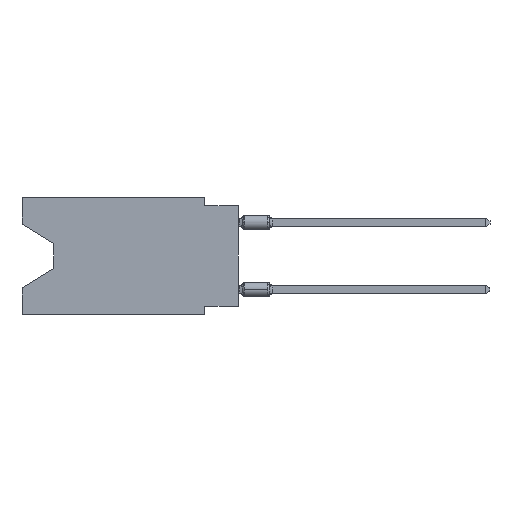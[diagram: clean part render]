
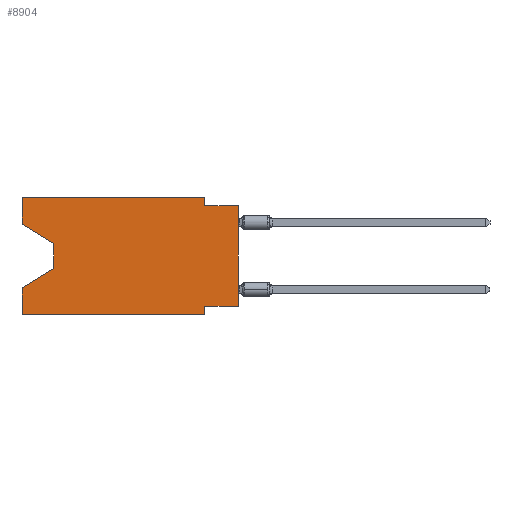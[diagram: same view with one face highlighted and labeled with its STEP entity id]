
A CAD part, left-side view. The second image highlights one B-rep face of the part: STEP entity #8904.
In plain terms, the highlighted planar face has unit normal (-1, 0, 0).
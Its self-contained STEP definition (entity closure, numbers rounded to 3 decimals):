
#585 = LINE ( 'NONE', #5144, #2630 ) ;
#1254 = EDGE_CURVE ( 'NONE', #11337, #13501, #20487, .T. ) ;
#1260 = EDGE_CURVE ( 'NONE', #18649, #28238, #6542, .T. ) ;
#2246 = EDGE_CURVE ( 'NONE', #20303, #17698, #585, .T. ) ;
#2630 = VECTOR ( 'NONE', #2946, 1000. ) ;
#2683 = VERTEX_POINT ( 'NONE', #18905 ) ;
#2846 = ORIENTED_EDGE ( 'NONE', *, *, #17076, .T. ) ;
#2946 = DIRECTION ( 'NONE',  ( 0., 0., 1. ) ) ;
#3536 = CARTESIAN_POINT ( 'NONE',  ( 0., 13.97, -3.505 ) ) ;
#3620 = VECTOR ( 'NONE', #18271, 1000. ) ;
#3776 = LINE ( 'NONE', #15995, #3787 ) ;
#3787 = VECTOR ( 'NONE', #20695, 1000. ) ;
#3843 = ORIENTED_EDGE ( 'NONE', *, *, #13008, .F. ) ;
#4056 = PLANE ( 'NONE',  #18541 ) ;
#5144 = CARTESIAN_POINT ( 'NONE',  ( 0., 16.383, 0. ) ) ;
#5709 = CARTESIAN_POINT ( 'NONE',  ( 0., 2.54, -8.89 ) ) ;
#5882 = CARTESIAN_POINT ( 'NONE',  ( 0., 16.383, -8.89 ) ) ;
#6039 = DIRECTION ( 'NONE',  ( 0., -1., 0. ) ) ;
#6542 = LINE ( 'NONE', #30690, #12105 ) ;
#6664 = LINE ( 'NONE', #25480, #3620 ) ;
#7456 = EDGE_CURVE ( 'NONE', #12397, #16086, #17240, .T. ) ;
#7503 = DIRECTION ( 'NONE',  ( 0., -1., 0. ) ) ;
#7618 = CARTESIAN_POINT ( 'NONE',  ( 0., 2.54, -8.255 ) ) ;
#7803 = DIRECTION ( 'NONE',  ( 0., 1., 0. ) ) ;
#8337 = CARTESIAN_POINT ( 'NONE',  ( 0., 0., -8.255 ) ) ;
#8385 = CARTESIAN_POINT ( 'NONE',  ( 0., 16.383, -2.038 ) ) ;
#8611 = LINE ( 'NONE', #29796, #20821 ) ;
#8904 = ADVANCED_FACE ( 'NONE', ( #23489 ), #4056, .F. ) ;
#10144 = CARTESIAN_POINT ( 'NONE',  ( 0., 0., -8.255 ) ) ;
#10667 = VERTEX_POINT ( 'NONE', #7618 ) ;
#10726 = DIRECTION ( 'NONE',  ( 0., 0., -1. ) ) ;
#10823 = DIRECTION ( 'NONE',  ( 0., 0., 1. ) ) ;
#10824 = EDGE_CURVE ( 'NONE', #28161, #13501, #24693, .T. ) ;
#10948 = EDGE_CURVE ( 'NONE', #28238, #28714, #6664, .T. ) ;
#11337 = VERTEX_POINT ( 'NONE', #8337 ) ;
#11439 = DIRECTION ( 'NONE',  ( 0., 0., -1. ) ) ;
#12105 = VECTOR ( 'NONE', #16103, 1000. ) ;
#12397 = VERTEX_POINT ( 'NONE', #30983 ) ;
#12553 = CARTESIAN_POINT ( 'NONE',  ( 0., 16.383, 0. ) ) ;
#12578 = ORIENTED_EDGE ( 'NONE', *, *, #13230, .F. ) ;
#12951 = CARTESIAN_POINT ( 'NONE',  ( 0., 2.54, -0.635 ) ) ;
#13008 = EDGE_CURVE ( 'NONE', #18649, #12397, #8611, .T. ) ;
#13088 = LINE ( 'NONE', #5709, #22534 ) ;
#13230 = EDGE_CURVE ( 'NONE', #11337, #10667, #17195, .T. ) ;
#13501 = VERTEX_POINT ( 'NONE', #20946 ) ;
#13663 = VECTOR ( 'NONE', #6039, 1000. ) ;
#14454 = EDGE_LOOP ( 'NONE', ( #15346, #22153, #16918, #21498, #2846, #15390, #12578, #14849, #19000, #14774, #26687, #3843 ) ) ;
#14774 = ORIENTED_EDGE ( 'NONE', *, *, #29946, .F. ) ;
#14849 = ORIENTED_EDGE ( 'NONE', *, *, #1254, .T. ) ;
#14976 = CARTESIAN_POINT ( 'NONE',  ( 0., 0., -0.635 ) ) ;
#15346 = ORIENTED_EDGE ( 'NONE', *, *, #1260, .T. ) ;
#15390 = ORIENTED_EDGE ( 'NONE', *, *, #23263, .F. ) ;
#15418 = LINE ( 'NONE', #22628, #27163 ) ;
#15995 = CARTESIAN_POINT ( 'NONE',  ( 0., 13.97, -5.385 ) ) ;
#16086 = VERTEX_POINT ( 'NONE', #18868 ) ;
#16103 = DIRECTION ( 'NONE',  ( 0., -0.855, -0.519 ) ) ;
#16647 = CARTESIAN_POINT ( 'NONE',  ( 0., 16.383, -6.852 ) ) ;
#16918 = ORIENTED_EDGE ( 'NONE', *, *, #17964, .T. ) ;
#17076 = EDGE_CURVE ( 'NONE', #20303, #2683, #28991, .T. ) ;
#17195 = LINE ( 'NONE', #10144, #27882 ) ;
#17240 = LINE ( 'NONE', #12553, #26232 ) ;
#17698 = VERTEX_POINT ( 'NONE', #16647 ) ;
#17964 = EDGE_CURVE ( 'NONE', #28714, #17698, #3776, .T. ) ;
#18271 = DIRECTION ( 'NONE',  ( 0., 0., -1. ) ) ;
#18541 = AXIS2_PLACEMENT_3D ( 'NONE', #28373, #26014, #11439 ) ;
#18649 = VERTEX_POINT ( 'NONE', #8385 ) ;
#18868 = CARTESIAN_POINT ( 'NONE',  ( 0., 2.54, 0. ) ) ;
#18905 = CARTESIAN_POINT ( 'NONE',  ( 0., 2.54, -8.89 ) ) ;
#19000 = ORIENTED_EDGE ( 'NONE', *, *, #10824, .F. ) ;
#19593 = VECTOR ( 'NONE', #28028, 1000. ) ;
#19966 = CARTESIAN_POINT ( 'NONE',  ( 0., 16.383, -8.89 ) ) ;
#20303 = VERTEX_POINT ( 'NONE', #19966 ) ;
#20487 = LINE ( 'NONE', #28341, #19593 ) ;
#20695 = DIRECTION ( 'NONE',  ( 0., 0.855, -0.519 ) ) ;
#20821 = VECTOR ( 'NONE', #10823, 1000. ) ;
#20946 = CARTESIAN_POINT ( 'NONE',  ( 0., 0., -0.635 ) ) ;
#21359 = CARTESIAN_POINT ( 'NONE',  ( 0., 13.97, -5.385 ) ) ;
#21498 = ORIENTED_EDGE ( 'NONE', *, *, #2246, .F. ) ;
#22153 = ORIENTED_EDGE ( 'NONE', *, *, #10948, .T. ) ;
#22534 = VECTOR ( 'NONE', #22641, 1000. ) ;
#22628 = CARTESIAN_POINT ( 'NONE',  ( 0., 2.54, 0. ) ) ;
#22641 = DIRECTION ( 'NONE',  ( 0., 0., -1. ) ) ;
#23263 = EDGE_CURVE ( 'NONE', #10667, #2683, #13088, .T. ) ;
#23489 = FACE_OUTER_BOUND ( 'NONE', #14454, .T. ) ;
#23764 = VECTOR ( 'NONE', #7503, 1000. ) ;
#24693 = LINE ( 'NONE', #14976, #13663 ) ;
#25480 = CARTESIAN_POINT ( 'NONE',  ( 0., 13.97, -3.505 ) ) ;
#26014 = DIRECTION ( 'NONE',  ( 1., 0., 0. ) ) ;
#26232 = VECTOR ( 'NONE', #26825, 1000. ) ;
#26687 = ORIENTED_EDGE ( 'NONE', *, *, #7456, .F. ) ;
#26825 = DIRECTION ( 'NONE',  ( 0., -1., 0. ) ) ;
#27163 = VECTOR ( 'NONE', #10726, 1000. ) ;
#27882 = VECTOR ( 'NONE', #7803, 1000. ) ;
#28028 = DIRECTION ( 'NONE',  ( 0., 0., 1. ) ) ;
#28161 = VERTEX_POINT ( 'NONE', #12951 ) ;
#28238 = VERTEX_POINT ( 'NONE', #3536 ) ;
#28341 = CARTESIAN_POINT ( 'NONE',  ( 0., 0., 0. ) ) ;
#28373 = CARTESIAN_POINT ( 'NONE',  ( 0., 16.383, 0. ) ) ;
#28714 = VERTEX_POINT ( 'NONE', #21359 ) ;
#28991 = LINE ( 'NONE', #5882, #23764 ) ;
#29796 = CARTESIAN_POINT ( 'NONE',  ( 0., 16.383, 0. ) ) ;
#29946 = EDGE_CURVE ( 'NONE', #16086, #28161, #15418, .T. ) ;
#30690 = CARTESIAN_POINT ( 'NONE',  ( 0., 16.383, -2.038 ) ) ;
#30983 = CARTESIAN_POINT ( 'NONE',  ( 0., 16.383, 0. ) ) ;
